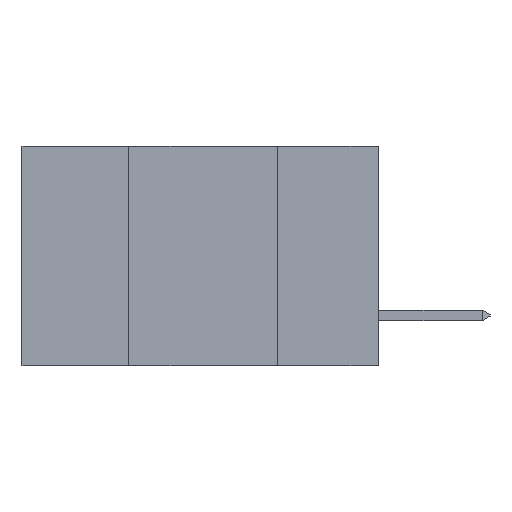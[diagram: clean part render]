
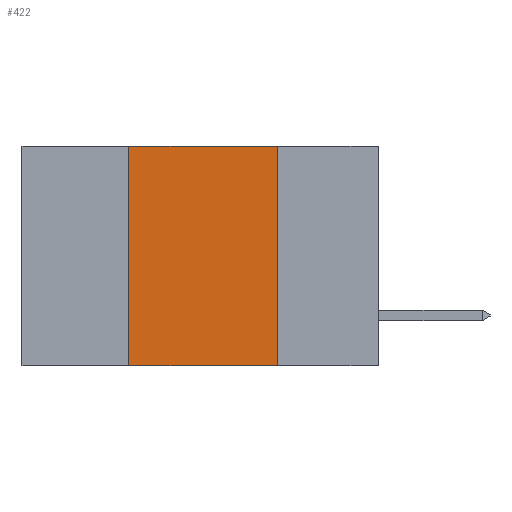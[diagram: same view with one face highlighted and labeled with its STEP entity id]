
A CAD part, left-side view. The second image highlights one B-rep face of the part: STEP entity #422.
In plain terms, the highlighted planar face has unit normal (-1, 0, 0).
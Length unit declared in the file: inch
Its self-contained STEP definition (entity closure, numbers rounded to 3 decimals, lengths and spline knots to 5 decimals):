
#15 = VERTEX_POINT ( 'NONE', #1365 ) ;
#21 = DIRECTION ( 'NONE',  ( 1., 0., 0. ) ) ;
#152 = VECTOR ( 'NONE', #1077, 39.37008 ) ;
#235 = VECTOR ( 'NONE', #3537, 39.37008 ) ;
#306 = DIRECTION ( 'NONE',  ( 0., 0., -1. ) ) ;
#352 = CARTESIAN_POINT ( 'NONE',  ( 0., 0.17, -0.37 ) ) ;
#422 = ADVANCED_FACE ( 'NONE', ( #3455 ), #957, .F. ) ;
#518 = VECTOR ( 'NONE', #1949, 39.37008 ) ;
#574 = DIRECTION ( 'NONE',  ( 0., 0., -1. ) ) ;
#604 = CARTESIAN_POINT ( 'NONE',  ( 0., 0.42, -0.37 ) ) ;
#856 = VERTEX_POINT ( 'NONE', #1566 ) ;
#957 = PLANE ( 'NONE',  #2231 ) ;
#985 = EDGE_CURVE ( 'NONE', #5023, #15, #4441, .T. ) ;
#1017 = CARTESIAN_POINT ( 'NONE',  ( 0., 0.6, 0. ) ) ;
#1077 = DIRECTION ( 'NONE',  ( 0., -1., 0. ) ) ;
#1235 = CARTESIAN_POINT ( 'NONE',  ( 0., 0.42, -0.37 ) ) ;
#1365 = CARTESIAN_POINT ( 'NONE',  ( 0., 0.17, -0.37 ) ) ;
#1510 = CARTESIAN_POINT ( 'NONE',  ( 0., 0.6, 0. ) ) ;
#1566 = CARTESIAN_POINT ( 'NONE',  ( 0., 0.42, 0. ) ) ;
#1949 = DIRECTION ( 'NONE',  ( 0., 0., 1. ) ) ;
#2148 = LINE ( 'NONE', #2969, #235 ) ;
#2231 = AXIS2_PLACEMENT_3D ( 'NONE', #1017, #21, #574 ) ;
#2265 = ORIENTED_EDGE ( 'NONE', *, *, #5034, .T. ) ;
#2439 = LINE ( 'NONE', #1235, #518 ) ;
#2840 = CARTESIAN_POINT ( 'NONE',  ( 0., 0.17, 0. ) ) ;
#2969 = CARTESIAN_POINT ( 'NONE',  ( 0., 0.6, -0.37 ) ) ;
#3175 = EDGE_LOOP ( 'NONE', ( #3536, #5045, #5807, #2265 ) ) ;
#3455 = FACE_OUTER_BOUND ( 'NONE', #3175, .T. ) ;
#3536 = ORIENTED_EDGE ( 'NONE', *, *, #985, .F. ) ;
#3537 = DIRECTION ( 'NONE',  ( 0., -1., 0. ) ) ;
#3759 = EDGE_CURVE ( 'NONE', #856, #5023, #7613, .T. ) ;
#4441 = LINE ( 'NONE', #352, #7877 ) ;
#4965 = VERTEX_POINT ( 'NONE', #604 ) ;
#5023 = VERTEX_POINT ( 'NONE', #2840 ) ;
#5034 = EDGE_CURVE ( 'NONE', #4965, #15, #2148, .T. ) ;
#5045 = ORIENTED_EDGE ( 'NONE', *, *, #3759, .F. ) ;
#5807 = ORIENTED_EDGE ( 'NONE', *, *, #8429, .F. ) ;
#7613 = LINE ( 'NONE', #1510, #152 ) ;
#7877 = VECTOR ( 'NONE', #306, 39.37008 ) ;
#8429 = EDGE_CURVE ( 'NONE', #4965, #856, #2439, .T. ) ;
